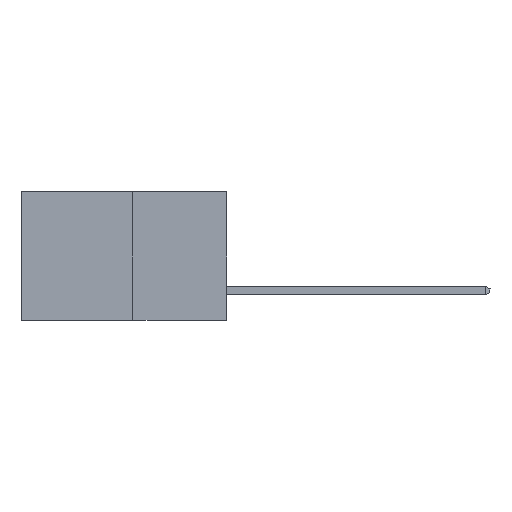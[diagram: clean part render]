
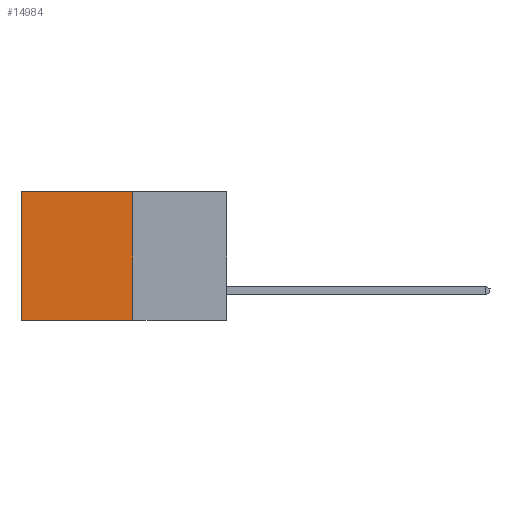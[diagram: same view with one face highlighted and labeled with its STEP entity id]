
A CAD part, left-side view. The second image highlights one B-rep face of the part: STEP entity #14984.
In plain terms, the highlighted planar face has unit normal (-1, 0, 0).
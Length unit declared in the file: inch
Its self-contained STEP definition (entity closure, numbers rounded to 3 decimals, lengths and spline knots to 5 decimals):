
#369 = EDGE_CURVE ( 'NONE', #12224, #14487, #6026, .T. ) ;
#414 = LINE ( 'NONE', #13272, #13723 ) ;
#616 = VECTOR ( 'NONE', #13939, 39.37008 ) ;
#1327 = EDGE_LOOP ( 'NONE', ( #4087, #4038, #4022, #3947 ) ) ;
#1581 = CARTESIAN_POINT ( 'NONE',  ( 0.277, 0.27, -0.37 ) ) ;
#2449 = DIRECTION ( 'NONE',  ( 1., 0., 0. ) ) ;
#3179 = EDGE_CURVE ( 'NONE', #14487, #5658, #4043, .T. ) ;
#3947 = ORIENTED_EDGE ( 'NONE', *, *, #9477, .T. ) ;
#4022 = ORIENTED_EDGE ( 'NONE', *, *, #369, .F. ) ;
#4038 = ORIENTED_EDGE ( 'NONE', *, *, #3179, .F. ) ;
#4043 = LINE ( 'NONE', #13967, #616 ) ;
#4087 = ORIENTED_EDGE ( 'NONE', *, *, #10977, .T. ) ;
#4415 = VERTEX_POINT ( 'NONE', #4512 ) ;
#4512 = CARTESIAN_POINT ( 'NONE',  ( 0.277, 0.59, 0. ) ) ;
#4894 = CARTESIAN_POINT ( 'NONE',  ( 0.277, 0.27, 0. ) ) ;
#5005 = CARTESIAN_POINT ( 'NONE',  ( 0.277, 0.27, 0. ) ) ;
#5152 = LINE ( 'NONE', #4894, #10942 ) ;
#5215 = CARTESIAN_POINT ( 'NONE',  ( 0.277, 0.27, -0.37 ) ) ;
#5658 = VERTEX_POINT ( 'NONE', #8098 ) ;
#6026 = LINE ( 'NONE', #15764, #8893 ) ;
#8098 = CARTESIAN_POINT ( 'NONE',  ( 0.277, 0.59, -0.37 ) ) ;
#8893 = VECTOR ( 'NONE', #15891, 39.37008 ) ;
#9477 = EDGE_CURVE ( 'NONE', #12224, #4415, #5152, .T. ) ;
#9830 = DIRECTION ( 'NONE',  ( 0., 1., 0. ) ) ;
#10942 = VECTOR ( 'NONE', #9830, 39.37008 ) ;
#10977 = EDGE_CURVE ( 'NONE', #4415, #5658, #414, .T. ) ;
#11388 = DIRECTION ( 'NONE',  ( 0., 0., -1. ) ) ;
#12224 = VERTEX_POINT ( 'NONE', #5005 ) ;
#13272 = CARTESIAN_POINT ( 'NONE',  ( 0.277, 0.59, -0.37 ) ) ;
#13723 = VECTOR ( 'NONE', #14414, 39.37008 ) ;
#13939 = DIRECTION ( 'NONE',  ( 0., 1., 0. ) ) ;
#13967 = CARTESIAN_POINT ( 'NONE',  ( 0.277, 0.27, -0.37 ) ) ;
#14414 = DIRECTION ( 'NONE',  ( 0., 0., -1. ) ) ;
#14487 = VERTEX_POINT ( 'NONE', #1581 ) ;
#14531 = FACE_OUTER_BOUND ( 'NONE', #1327, .T. ) ;
#14984 = ADVANCED_FACE ( 'NONE', ( #14531 ), #16051, .F. ) ;
#15075 = AXIS2_PLACEMENT_3D ( 'NONE', #5215, #2449, #11388 ) ;
#15764 = CARTESIAN_POINT ( 'NONE',  ( 0.277, 0.27, -0.37 ) ) ;
#15891 = DIRECTION ( 'NONE',  ( 0., 0., -1. ) ) ;
#16051 = PLANE ( 'NONE',  #15075 ) ;
